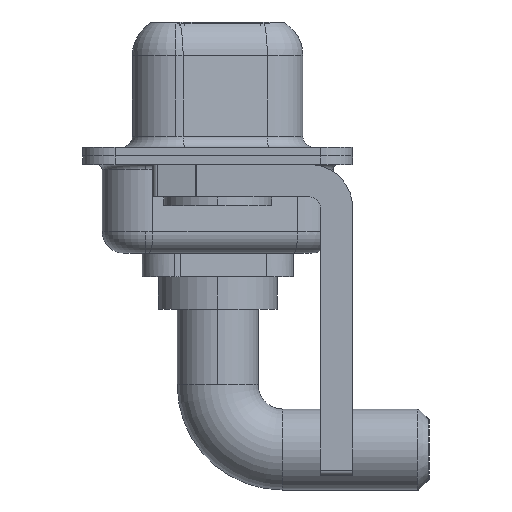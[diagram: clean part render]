
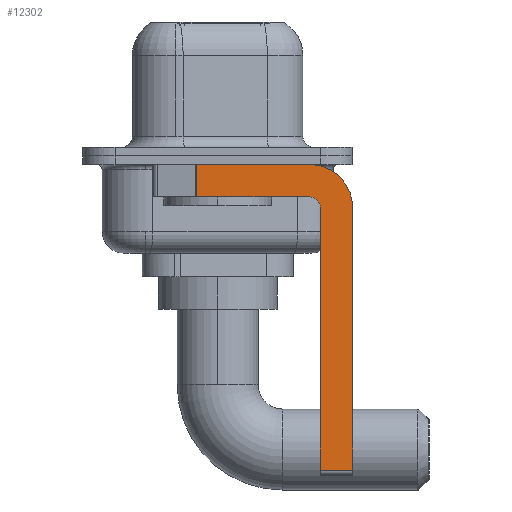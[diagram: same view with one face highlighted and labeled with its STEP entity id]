
A CAD part, left-side view. The second image highlights one B-rep face of the part: STEP entity #12302.
In plain terms, the highlighted planar face has unit normal (-1, 0, 0).
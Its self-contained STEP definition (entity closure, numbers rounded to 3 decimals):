
#201 = AXIS2_PLACEMENT_3D ( 'NONE', #12060, #8344, #12877 ) ;
#210 = CIRCLE ( 'NONE', #201, 2. ) ;
#1107 = CARTESIAN_POINT ( 'NONE',  ( -2.9, -4.25, -14.55 ) ) ;
#1124 = ORIENTED_EDGE ( 'NONE', *, *, #2316, .F. ) ;
#1130 = CARTESIAN_POINT ( 'NONE',  ( -2.9, -4.75, -14.55 ) ) ;
#1187 = CARTESIAN_POINT ( 'NONE',  ( -2.9, -6.25, -14.55 ) ) ;
#1281 = EDGE_CURVE ( 'NONE', #5675, #2187, #7498, .T. ) ;
#1623 = CARTESIAN_POINT ( 'NONE',  ( -2.9, 0.978, -0.4 ) ) ;
#1908 = CARTESIAN_POINT ( 'NONE',  ( -2.9, -4.75, -14.8 ) ) ;
#2020 = VERTEX_POINT ( 'NONE', #13612 ) ;
#2187 = VERTEX_POINT ( 'NONE', #7392 ) ;
#2272 = EDGE_CURVE ( 'NONE', #2187, #2020, #13856, .T. ) ;
#2316 = EDGE_CURVE ( 'NONE', #4440, #3367, #210, .T. ) ;
#2586 = CARTESIAN_POINT ( 'NONE',  ( -2.9, 0.978, -1.9 ) ) ;
#2904 = DIRECTION ( 'NONE',  ( -1., 0., 0. ) ) ;
#3367 = VERTEX_POINT ( 'NONE', #9516 ) ;
#3572 = FACE_OUTER_BOUND ( 'NONE', #11000, .T. ) ;
#3675 = EDGE_CURVE ( 'NONE', #3897, #14498, #13873, .T. ) ;
#3863 = PLANE ( 'NONE',  #4116 ) ;
#3897 = VERTEX_POINT ( 'NONE', #1623 ) ;
#4116 = AXIS2_PLACEMENT_3D ( 'NONE', #12637, #13981, #4749 ) ;
#4188 = DIRECTION ( 'NONE',  ( 0., 0., 1. ) ) ;
#4440 = VERTEX_POINT ( 'NONE', #4985 ) ;
#4749 = DIRECTION ( 'NONE',  ( 0., 0., -1. ) ) ;
#4985 = CARTESIAN_POINT ( 'NONE',  ( -2.9, -4.25, -0.4 ) ) ;
#5119 = EDGE_CURVE ( 'NONE', #3897, #4440, #10326, .T. ) ;
#5165 = VECTOR ( 'NONE', #13796, 1000. ) ;
#5339 = CARTESIAN_POINT ( 'NONE',  ( -2.9, -4.25, -2.4 ) ) ;
#5439 = ORIENTED_EDGE ( 'NONE', *, *, #10401, .F. ) ;
#5675 = VERTEX_POINT ( 'NONE', #1130 ) ;
#6184 = DIRECTION ( 'NONE',  ( 0., 0., -1. ) ) ;
#6313 = ORIENTED_EDGE ( 'NONE', *, *, #5119, .F. ) ;
#7027 = VECTOR ( 'NONE', #11447, 1000. ) ;
#7392 = CARTESIAN_POINT ( 'NONE',  ( -2.9, -4.75, -2.4 ) ) ;
#7498 = LINE ( 'NONE', #1908, #10151 ) ;
#8344 = DIRECTION ( 'NONE',  ( 1., 0., 0. ) ) ;
#9361 = AXIS2_PLACEMENT_3D ( 'NONE', #5339, #2904, #14278 ) ;
#9432 = LINE ( 'NONE', #11814, #13294 ) ;
#9516 = CARTESIAN_POINT ( 'NONE',  ( -2.9, -6.25, -2.4 ) ) ;
#9522 = VECTOR ( 'NONE', #13347, 1000. ) ;
#9927 = DIRECTION ( 'NONE',  ( 0., 1., 0. ) ) ;
#10151 = VECTOR ( 'NONE', #4188, 1000. ) ;
#10326 = LINE ( 'NONE', #12554, #7027 ) ;
#10401 = EDGE_CURVE ( 'NONE', #2020, #14498, #13345, .T. ) ;
#10982 = ORIENTED_EDGE ( 'NONE', *, *, #1281, .F. ) ;
#11000 = EDGE_LOOP ( 'NONE', ( #6313, #14435, #5439, #13897, #10982, #13387, #12986, #1124 ) ) ;
#11039 = EDGE_CURVE ( 'NONE', #3367, #13714, #9432, .T. ) ;
#11148 = CARTESIAN_POINT ( 'NONE',  ( -2.9, 0.978, -1.9 ) ) ;
#11187 = LINE ( 'NONE', #1107, #9522 ) ;
#11257 = CARTESIAN_POINT ( 'NONE',  ( -2.9, -4.25, -1.9 ) ) ;
#11447 = DIRECTION ( 'NONE',  ( 0., -1., 0. ) ) ;
#11800 = EDGE_CURVE ( 'NONE', #5675, #13714, #11187, .T. ) ;
#11814 = CARTESIAN_POINT ( 'NONE',  ( -2.9, -6.25, -2.4 ) ) ;
#12060 = CARTESIAN_POINT ( 'NONE',  ( -2.9, -4.25, -2.4 ) ) ;
#12137 = VECTOR ( 'NONE', #9927, 1000. ) ;
#12302 = ADVANCED_FACE ( 'NONE', ( #3572 ), #3863, .F. ) ;
#12554 = CARTESIAN_POINT ( 'NONE',  ( -2.9, 3., -0.4 ) ) ;
#12637 = CARTESIAN_POINT ( 'NONE',  ( -2.9, -4.25, -2.4 ) ) ;
#12877 = DIRECTION ( 'NONE',  ( 0., 0., -1. ) ) ;
#12986 = ORIENTED_EDGE ( 'NONE', *, *, #11039, .F. ) ;
#13294 = VECTOR ( 'NONE', #6184, 1000. ) ;
#13345 = LINE ( 'NONE', #11257, #12137 ) ;
#13347 = DIRECTION ( 'NONE',  ( 0., -1., 0. ) ) ;
#13387 = ORIENTED_EDGE ( 'NONE', *, *, #11800, .T. ) ;
#13612 = CARTESIAN_POINT ( 'NONE',  ( -2.9, -4.25, -1.9 ) ) ;
#13714 = VERTEX_POINT ( 'NONE', #1187 ) ;
#13796 = DIRECTION ( 'NONE',  ( 0., 0., -1. ) ) ;
#13856 = CIRCLE ( 'NONE', #9361, 0.5 ) ;
#13873 = LINE ( 'NONE', #2586, #5165 ) ;
#13897 = ORIENTED_EDGE ( 'NONE', *, *, #2272, .F. ) ;
#13981 = DIRECTION ( 'NONE',  ( 1., 0., 0. ) ) ;
#14278 = DIRECTION ( 'NONE',  ( 0., 0., 1. ) ) ;
#14435 = ORIENTED_EDGE ( 'NONE', *, *, #3675, .T. ) ;
#14498 = VERTEX_POINT ( 'NONE', #11148 ) ;
